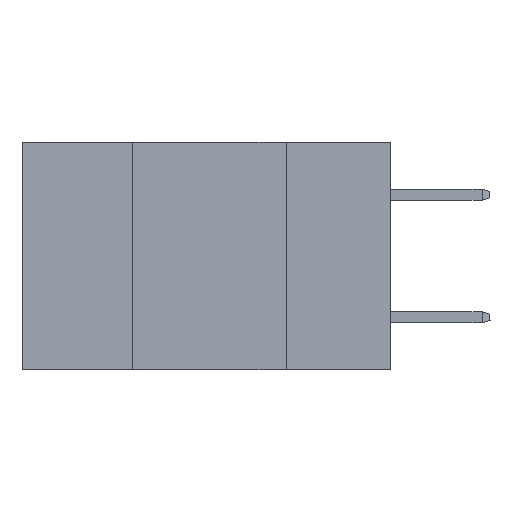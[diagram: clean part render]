
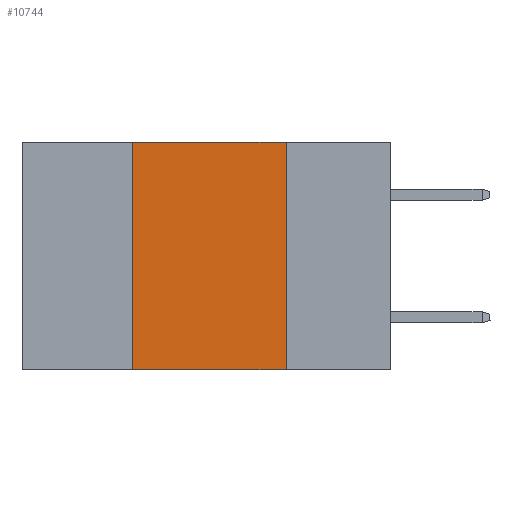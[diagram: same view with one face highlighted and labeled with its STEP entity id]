
A CAD part, left-side view. The second image highlights one B-rep face of the part: STEP entity #10744.
In plain terms, the highlighted planar face has unit normal (-1, 0, 0).
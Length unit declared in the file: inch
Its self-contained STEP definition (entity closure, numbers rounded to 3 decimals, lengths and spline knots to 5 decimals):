
#31 = VERTEX_POINT ( 'NONE', #865 ) ;
#175 = VERTEX_POINT ( 'NONE', #11514 ) ;
#865 = CARTESIAN_POINT ( 'NONE',  ( 0., 0.42, 0. ) ) ;
#1434 = LINE ( 'NONE', #9610, #1997 ) ;
#1469 = EDGE_CURVE ( 'NONE', #31, #11868, #2699, .T. ) ;
#1497 = ORIENTED_EDGE ( 'NONE', *, *, #12255, .F. ) ;
#1997 = VECTOR ( 'NONE', #7660, 39.37008 ) ;
#2362 = DIRECTION ( 'NONE',  ( 0., -1., 0. ) ) ;
#2457 = ORIENTED_EDGE ( 'NONE', *, *, #4527, .F. ) ;
#2699 = LINE ( 'NONE', #12378, #6779 ) ;
#2831 = DIRECTION ( 'NONE',  ( 0., 0., 1. ) ) ;
#4123 = EDGE_CURVE ( 'NONE', #9255, #175, #7000, .T. ) ;
#4382 = CARTESIAN_POINT ( 'NONE',  ( 0., 0.6, 0. ) ) ;
#4527 = EDGE_CURVE ( 'NONE', #9255, #31, #7764, .T. ) ;
#5621 = CARTESIAN_POINT ( 'NONE',  ( 0., 0.17, 0. ) ) ;
#5845 = ORIENTED_EDGE ( 'NONE', *, *, #4123, .T. ) ;
#5944 = VECTOR ( 'NONE', #2831, 39.37008 ) ;
#6210 = DIRECTION ( 'NONE',  ( 1., 0., 0. ) ) ;
#6779 = VECTOR ( 'NONE', #7590, 39.37008 ) ;
#6908 = FACE_OUTER_BOUND ( 'NONE', #11587, .T. ) ;
#7000 = LINE ( 'NONE', #8031, #10450 ) ;
#7236 = CARTESIAN_POINT ( 'NONE',  ( 0., 0.42, -0.37 ) ) ;
#7590 = DIRECTION ( 'NONE',  ( 0., -1., 0. ) ) ;
#7645 = ORIENTED_EDGE ( 'NONE', *, *, #1469, .F. ) ;
#7660 = DIRECTION ( 'NONE',  ( 0., 0., -1. ) ) ;
#7764 = LINE ( 'NONE', #9414, #5944 ) ;
#8031 = CARTESIAN_POINT ( 'NONE',  ( 0., 0.6, -0.37 ) ) ;
#8102 = AXIS2_PLACEMENT_3D ( 'NONE', #4382, #6210, #11075 ) ;
#9135 = PLANE ( 'NONE',  #8102 ) ;
#9255 = VERTEX_POINT ( 'NONE', #7236 ) ;
#9414 = CARTESIAN_POINT ( 'NONE',  ( 0., 0.42, 0. ) ) ;
#9610 = CARTESIAN_POINT ( 'NONE',  ( 0., 0.17, 0. ) ) ;
#10450 = VECTOR ( 'NONE', #2362, 39.37008 ) ;
#10744 = ADVANCED_FACE ( 'NONE', ( #6908 ), #9135, .F. ) ;
#11075 = DIRECTION ( 'NONE',  ( 0., 0., -1. ) ) ;
#11514 = CARTESIAN_POINT ( 'NONE',  ( 0., 0.17, -0.37 ) ) ;
#11587 = EDGE_LOOP ( 'NONE', ( #1497, #7645, #2457, #5845 ) ) ;
#11868 = VERTEX_POINT ( 'NONE', #5621 ) ;
#12255 = EDGE_CURVE ( 'NONE', #11868, #175, #1434, .T. ) ;
#12378 = CARTESIAN_POINT ( 'NONE',  ( 0., 0.6, 0. ) ) ;
